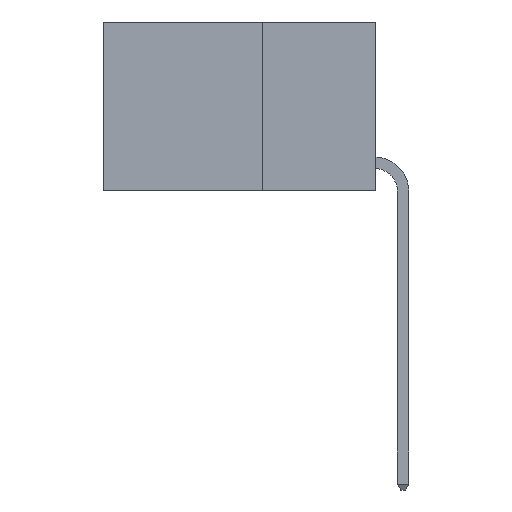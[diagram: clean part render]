
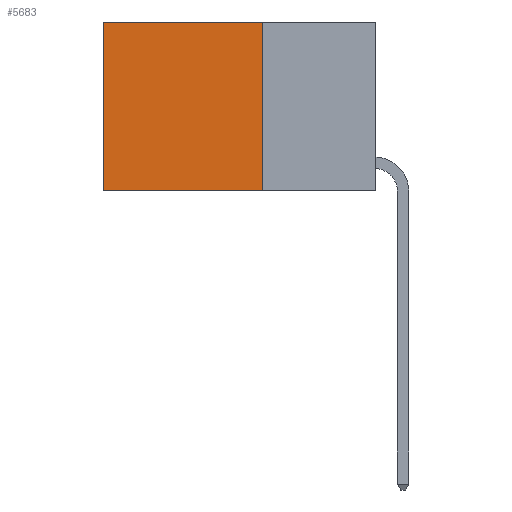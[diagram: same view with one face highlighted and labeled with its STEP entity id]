
A CAD part, left-side view. The second image highlights one B-rep face of the part: STEP entity #5683.
In plain terms, the highlighted planar face has unit normal (-1, 0, 0).
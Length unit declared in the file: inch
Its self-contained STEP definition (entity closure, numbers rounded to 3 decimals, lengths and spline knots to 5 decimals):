
#124 = DIRECTION ( 'NONE',  ( 0., 1., 0. ) ) ;
#609 = CARTESIAN_POINT ( 'NONE',  ( 0.2625, 0.25, 0. ) ) ;
#1409 = CARTESIAN_POINT ( 'NONE',  ( 0.2625, 0.6, 0. ) ) ;
#1479 = EDGE_CURVE ( 'NONE', #5505, #1558, #9422, .T. ) ;
#1547 = VERTEX_POINT ( 'NONE', #5802 ) ;
#1558 = VERTEX_POINT ( 'NONE', #9365 ) ;
#1858 = EDGE_CURVE ( 'NONE', #1558, #8461, #6042, .T. ) ;
#2381 = CARTESIAN_POINT ( 'NONE',  ( 0.2625, 0.6, -0.37 ) ) ;
#2745 = VECTOR ( 'NONE', #3349, 39.37008 ) ;
#3311 = DIRECTION ( 'NONE',  ( 0., 0., -1. ) ) ;
#3349 = DIRECTION ( 'NONE',  ( 0., 0., -1. ) ) ;
#3598 = DIRECTION ( 'NONE',  ( 0., 1., 0. ) ) ;
#4822 = FACE_OUTER_BOUND ( 'NONE', #10546, .T. ) ;
#5083 = CARTESIAN_POINT ( 'NONE',  ( 0.2625, 0.25, 0. ) ) ;
#5505 = VERTEX_POINT ( 'NONE', #9867 ) ;
#5620 = AXIS2_PLACEMENT_3D ( 'NONE', #5083, #8560, #3311 ) ;
#5683 = ADVANCED_FACE ( 'NONE', ( #4822 ), #7736, .F. ) ;
#5802 = CARTESIAN_POINT ( 'NONE',  ( 0.2625, 0.25, -0.37 ) ) ;
#5969 = VECTOR ( 'NONE', #6128, 39.37008 ) ;
#6042 = LINE ( 'NONE', #1409, #5969 ) ;
#6128 = DIRECTION ( 'NONE',  ( 0., 0., -1. ) ) ;
#6201 = ORIENTED_EDGE ( 'NONE', *, *, #1858, .T. ) ;
#6537 = ORIENTED_EDGE ( 'NONE', *, *, #10358, .F. ) ;
#6643 = ORIENTED_EDGE ( 'NONE', *, *, #10822, .F. ) ;
#6684 = ORIENTED_EDGE ( 'NONE', *, *, #1479, .T. ) ;
#7736 = PLANE ( 'NONE',  #5620 ) ;
#7994 = CARTESIAN_POINT ( 'NONE',  ( 0.2625, 0.25, -0.37 ) ) ;
#8461 = VERTEX_POINT ( 'NONE', #2381 ) ;
#8542 = VECTOR ( 'NONE', #3598, 39.37008 ) ;
#8560 = DIRECTION ( 'NONE',  ( 1., 0., 0. ) ) ;
#8589 = CARTESIAN_POINT ( 'NONE',  ( 0.2625, 0.25, 0. ) ) ;
#8816 = LINE ( 'NONE', #7994, #8542 ) ;
#9174 = VECTOR ( 'NONE', #124, 39.37008 ) ;
#9365 = CARTESIAN_POINT ( 'NONE',  ( 0.2625, 0.6, 0. ) ) ;
#9422 = LINE ( 'NONE', #609, #9174 ) ;
#9444 = LINE ( 'NONE', #8589, #2745 ) ;
#9867 = CARTESIAN_POINT ( 'NONE',  ( 0.2625, 0.25, 0. ) ) ;
#10358 = EDGE_CURVE ( 'NONE', #1547, #8461, #8816, .T. ) ;
#10546 = EDGE_LOOP ( 'NONE', ( #6201, #6537, #6643, #6684 ) ) ;
#10822 = EDGE_CURVE ( 'NONE', #5505, #1547, #9444, .T. ) ;
